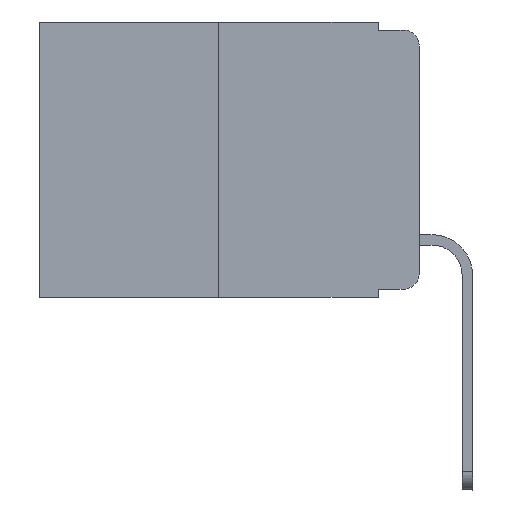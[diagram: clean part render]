
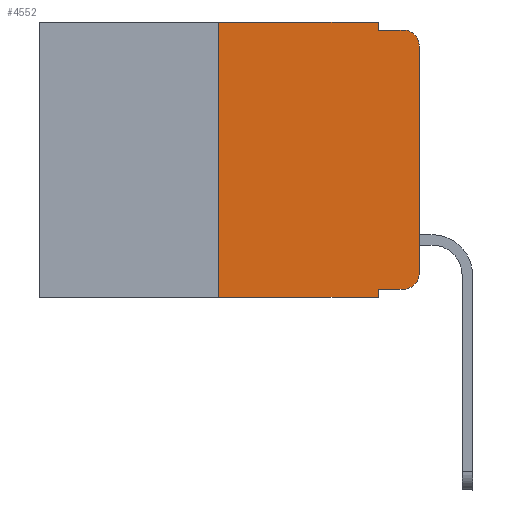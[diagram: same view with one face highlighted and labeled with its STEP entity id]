
A CAD part, left-side view. The second image highlights one B-rep face of the part: STEP entity #4552.
In plain terms, the highlighted planar face has unit normal (-1, 0, 0).
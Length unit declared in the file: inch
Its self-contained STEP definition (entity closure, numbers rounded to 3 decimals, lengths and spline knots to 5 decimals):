
#31 = ORIENTED_EDGE ( 'NONE', *, *, #9557, .F. ) ;
#52 = VERTEX_POINT ( 'NONE', #6840 ) ;
#224 = LINE ( 'NONE', #1600, #3329 ) ;
#452 = LINE ( 'NONE', #16126, #2243 ) ;
#733 = EDGE_CURVE ( 'NONE', #9487, #16304, #452, .T. ) ;
#1390 = AXIS2_PLACEMENT_3D ( 'NONE', #16579, #6398, #6310 ) ;
#1436 = ORIENTED_EDGE ( 'NONE', *, *, #8118, .T. ) ;
#1479 = EDGE_CURVE ( 'NONE', #5676, #1739, #16157, .T. ) ;
#1600 = CARTESIAN_POINT ( 'NONE',  ( 0., 0.051, -0.01 ) ) ;
#1739 = VERTEX_POINT ( 'NONE', #14581 ) ;
#1887 = CARTESIAN_POINT ( 'NONE',  ( 0., 0.02, -0.313 ) ) ;
#1936 = DIRECTION ( 'NONE',  ( 0., -1., 0. ) ) ;
#1979 = DIRECTION ( 'NONE',  ( 0., 0., -1. ) ) ;
#2133 = CARTESIAN_POINT ( 'NONE',  ( 0., 0.25, 0. ) ) ;
#2147 = CIRCLE ( 'NONE', #14802, 0.02 ) ;
#2241 = CARTESIAN_POINT ( 'NONE',  ( 0., 0.051, -0.01 ) ) ;
#2243 = VECTOR ( 'NONE', #4585, 39.37008 ) ;
#2343 = DIRECTION ( 'NONE',  ( 0., -1., 0. ) ) ;
#2438 = PLANE ( 'NONE',  #1390 ) ;
#2808 = VERTEX_POINT ( 'NONE', #16253 ) ;
#3329 = VECTOR ( 'NONE', #11868, 39.37008 ) ;
#4175 = EDGE_CURVE ( 'NONE', #5676, #52, #7229, .T. ) ;
#4481 = DIRECTION ( 'NONE',  ( 0., 0., 1. ) ) ;
#4515 = ORIENTED_EDGE ( 'NONE', *, *, #4175, .F. ) ;
#4552 = ADVANCED_FACE ( 'NONE', ( #4864 ), #2438, .F. ) ;
#4585 = DIRECTION ( 'NONE',  ( 0., 0., -1. ) ) ;
#4837 = CARTESIAN_POINT ( 'NONE',  ( 0., 0.02, -0.01 ) ) ;
#4864 = FACE_OUTER_BOUND ( 'NONE', #6035, .T. ) ;
#5676 = VERTEX_POINT ( 'NONE', #5939 ) ;
#5796 = CARTESIAN_POINT ( 'NONE',  ( 0., 0.473, -0.343 ) ) ;
#5875 = LINE ( 'NONE', #5796, #15823 ) ;
#5939 = CARTESIAN_POINT ( 'NONE',  ( 0., 0.051, -0.333 ) ) ;
#5953 = ORIENTED_EDGE ( 'NONE', *, *, #733, .F. ) ;
#5987 = ORIENTED_EDGE ( 'NONE', *, *, #10403, .T. ) ;
#6035 = EDGE_LOOP ( 'NONE', ( #5987, #6834, #14567, #5953, #31, #16206, #1436, #4515, #16757, #9712 ) ) ;
#6183 = EDGE_CURVE ( 'NONE', #11509, #16303, #8509, .T. ) ;
#6310 = DIRECTION ( 'NONE',  ( 0., 0., -1. ) ) ;
#6398 = DIRECTION ( 'NONE',  ( 1., 0., 0. ) ) ;
#6666 = EDGE_CURVE ( 'NONE', #1739, #11050, #2147, .T. ) ;
#6834 = ORIENTED_EDGE ( 'NONE', *, *, #6183, .T. ) ;
#6840 = CARTESIAN_POINT ( 'NONE',  ( 0., 0.051, -0.343 ) ) ;
#7229 = LINE ( 'NONE', #11183, #13078 ) ;
#8029 = LINE ( 'NONE', #13279, #12669 ) ;
#8118 = EDGE_CURVE ( 'NONE', #16732, #52, #5875, .T. ) ;
#8248 = VECTOR ( 'NONE', #15827, 39.37008 ) ;
#8509 = CIRCLE ( 'NONE', #10693, 0.02 ) ;
#9130 = CARTESIAN_POINT ( 'NONE',  ( 0., 0., -0.03 ) ) ;
#9487 = VERTEX_POINT ( 'NONE', #10786 ) ;
#9557 = EDGE_CURVE ( 'NONE', #2808, #9487, #8029, .T. ) ;
#9712 = ORIENTED_EDGE ( 'NONE', *, *, #6666, .T. ) ;
#9786 = CARTESIAN_POINT ( 'NONE',  ( 0., 0.051, -0.333 ) ) ;
#9904 = LINE ( 'NONE', #2133, #10754 ) ;
#9987 = DIRECTION ( 'NONE',  ( 0., 0., -1. ) ) ;
#10134 = EDGE_CURVE ( 'NONE', #16732, #2808, #9904, .T. ) ;
#10328 = EDGE_CURVE ( 'NONE', #16304, #16303, #224, .T. ) ;
#10403 = EDGE_CURVE ( 'NONE', #11050, #11509, #14617, .T. ) ;
#10693 = AXIS2_PLACEMENT_3D ( 'NONE', #12892, #14438, #16860 ) ;
#10754 = VECTOR ( 'NONE', #4481, 39.37008 ) ;
#10786 = CARTESIAN_POINT ( 'NONE',  ( 0., 0.051, 0. ) ) ;
#11030 = DIRECTION ( 'NONE',  ( -1., 0., 0. ) ) ;
#11050 = VERTEX_POINT ( 'NONE', #15363 ) ;
#11183 = CARTESIAN_POINT ( 'NONE',  ( 0., 0.051, 0. ) ) ;
#11509 = VERTEX_POINT ( 'NONE', #9130 ) ;
#11868 = DIRECTION ( 'NONE',  ( 0., -1., 0. ) ) ;
#12669 = VECTOR ( 'NONE', #15949, 39.37008 ) ;
#12892 = CARTESIAN_POINT ( 'NONE',  ( 0., 0.02, -0.03 ) ) ;
#13078 = VECTOR ( 'NONE', #9987, 39.37008 ) ;
#13279 = CARTESIAN_POINT ( 'NONE',  ( 0., 0.473, 0. ) ) ;
#13499 = CARTESIAN_POINT ( 'NONE',  ( 0., 0., 0. ) ) ;
#13991 = CARTESIAN_POINT ( 'NONE',  ( 0., 0.25, -0.343 ) ) ;
#14438 = DIRECTION ( 'NONE',  ( -1., 0., 0. ) ) ;
#14567 = ORIENTED_EDGE ( 'NONE', *, *, #10328, .F. ) ;
#14581 = CARTESIAN_POINT ( 'NONE',  ( 0., 0.02, -0.333 ) ) ;
#14617 = LINE ( 'NONE', #13499, #8248 ) ;
#14802 = AXIS2_PLACEMENT_3D ( 'NONE', #1887, #11030, #1979 ) ;
#15363 = CARTESIAN_POINT ( 'NONE',  ( 0., 0., -0.313 ) ) ;
#15430 = VECTOR ( 'NONE', #1936, 39.37008 ) ;
#15823 = VECTOR ( 'NONE', #2343, 39.37008 ) ;
#15827 = DIRECTION ( 'NONE',  ( 0., 0., 1. ) ) ;
#15949 = DIRECTION ( 'NONE',  ( 0., -1., 0. ) ) ;
#16126 = CARTESIAN_POINT ( 'NONE',  ( 0., 0.051, 0. ) ) ;
#16157 = LINE ( 'NONE', #9786, #15430 ) ;
#16206 = ORIENTED_EDGE ( 'NONE', *, *, #10134, .F. ) ;
#16253 = CARTESIAN_POINT ( 'NONE',  ( 0., 0.25, 0. ) ) ;
#16303 = VERTEX_POINT ( 'NONE', #4837 ) ;
#16304 = VERTEX_POINT ( 'NONE', #2241 ) ;
#16579 = CARTESIAN_POINT ( 'NONE',  ( 0., 0.473, 0. ) ) ;
#16732 = VERTEX_POINT ( 'NONE', #13991 ) ;
#16757 = ORIENTED_EDGE ( 'NONE', *, *, #1479, .T. ) ;
#16860 = DIRECTION ( 'NONE',  ( 0., 0., -1. ) ) ;
